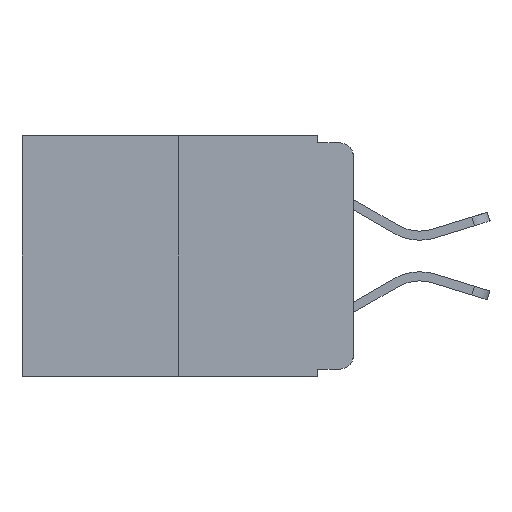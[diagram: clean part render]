
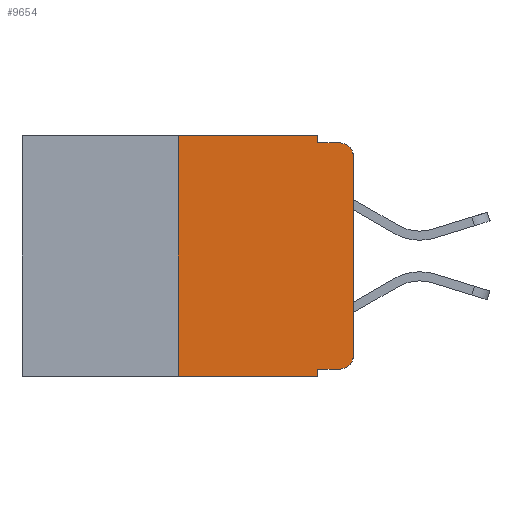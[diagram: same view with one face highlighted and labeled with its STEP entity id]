
A CAD part, left-side view. The second image highlights one B-rep face of the part: STEP entity #9654.
In plain terms, the highlighted planar face has unit normal (-1, 0, 0).
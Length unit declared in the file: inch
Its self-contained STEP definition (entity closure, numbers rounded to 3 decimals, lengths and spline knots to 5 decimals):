
#109 = ORIENTED_EDGE ( 'NONE', *, *, #12100, .F. ) ;
#621 = ORIENTED_EDGE ( 'NONE', *, *, #23641, .F. ) ;
#815 = LINE ( 'NONE', #3153, #20072 ) ;
#1207 = ORIENTED_EDGE ( 'NONE', *, *, #16410, .F. ) ;
#1382 = ORIENTED_EDGE ( 'NONE', *, *, #4426, .T. ) ;
#1397 = CARTESIAN_POINT ( 'NONE',  ( 0., 0.02, -0.03 ) ) ;
#1528 = CARTESIAN_POINT ( 'NONE',  ( 0., 0.051, -0.01 ) ) ;
#1575 = PLANE ( 'NONE',  #7291 ) ;
#1673 = ORIENTED_EDGE ( 'NONE', *, *, #8745, .F. ) ;
#1762 = CIRCLE ( 'NONE', #21992, 0.02 ) ;
#1882 = VECTOR ( 'NONE', #16348, 39.37008 ) ;
#2159 = ORIENTED_EDGE ( 'NONE', *, *, #24383, .T. ) ;
#2772 = ORIENTED_EDGE ( 'NONE', *, *, #15615, .T. ) ;
#3153 = CARTESIAN_POINT ( 'NONE',  ( 0., 0., 0. ) ) ;
#3206 = LINE ( 'NONE', #22989, #22865 ) ;
#3337 = ORIENTED_EDGE ( 'NONE', *, *, #15472, .T. ) ;
#3418 = DIRECTION ( 'NONE',  ( 0., 0., -1. ) ) ;
#3489 = ORIENTED_EDGE ( 'NONE', *, *, #11644, .T. ) ;
#4426 = EDGE_CURVE ( 'NONE', #17896, #7788, #3206, .T. ) ;
#4738 = DIRECTION ( 'NONE',  ( 0., 0., -1. ) ) ;
#5525 = CARTESIAN_POINT ( 'NONE',  ( 0., 0.473, 0. ) ) ;
#5597 = VERTEX_POINT ( 'NONE', #15322 ) ;
#6292 = VERTEX_POINT ( 'NONE', #21320 ) ;
#7291 = AXIS2_PLACEMENT_3D ( 'NONE', #5525, #24467, #13225 ) ;
#7560 = CARTESIAN_POINT ( 'NONE',  ( 0., 0.473, 0. ) ) ;
#7784 = LINE ( 'NONE', #8621, #17892 ) ;
#7788 = VERTEX_POINT ( 'NONE', #19120 ) ;
#7796 = EDGE_CURVE ( 'NONE', #18783, #20367, #13653, .T. ) ;
#7810 = CARTESIAN_POINT ( 'NONE',  ( 0., 0.051, -0.01 ) ) ;
#8621 = CARTESIAN_POINT ( 'NONE',  ( 0., 0.051, 0. ) ) ;
#8745 = EDGE_CURVE ( 'NONE', #5597, #7788, #17229, .T. ) ;
#9654 = ADVANCED_FACE ( 'NONE', ( #13890 ), #1575, .F. ) ;
#9754 = CARTESIAN_POINT ( 'NONE',  ( 0., 0.02, -0.313 ) ) ;
#9822 = DIRECTION ( 'NONE',  ( 0., -1., 0. ) ) ;
#9935 = EDGE_LOOP ( 'NONE', ( #3337, #3489, #10934, #109, #621, #1207, #1382, #1673, #2159, #2772 ) ) ;
#10069 = CARTESIAN_POINT ( 'NONE',  ( 0., 0.02, -0.01 ) ) ;
#10619 = CARTESIAN_POINT ( 'NONE',  ( 0., 0.051, 0. ) ) ;
#10934 = ORIENTED_EDGE ( 'NONE', *, *, #7796, .F. ) ;
#11644 = EDGE_CURVE ( 'NONE', #23990, #20367, #18529, .T. ) ;
#11646 = DIRECTION ( 'NONE',  ( 0., 0., -1. ) ) ;
#11850 = VECTOR ( 'NONE', #20224, 39.37008 ) ;
#12008 = DIRECTION ( 'NONE',  ( 0., 0., 1. ) ) ;
#12100 = EDGE_CURVE ( 'NONE', #13400, #18783, #7784, .T. ) ;
#13100 = CARTESIAN_POINT ( 'NONE',  ( 0., 0.25, -0.343 ) ) ;
#13225 = DIRECTION ( 'NONE',  ( 0., 0., -1. ) ) ;
#13342 = CARTESIAN_POINT ( 'NONE',  ( 0., 0., -0.313 ) ) ;
#13400 = VERTEX_POINT ( 'NONE', #24643 ) ;
#13653 = LINE ( 'NONE', #7810, #18726 ) ;
#13678 = CARTESIAN_POINT ( 'NONE',  ( 0., 0.02, -0.333 ) ) ;
#13890 = FACE_OUTER_BOUND ( 'NONE', #9935, .T. ) ;
#14921 = DIRECTION ( 'NONE',  ( -1., 0., 0. ) ) ;
#15172 = VECTOR ( 'NONE', #12008, 39.37008 ) ;
#15322 = CARTESIAN_POINT ( 'NONE',  ( 0., 0.051, -0.333 ) ) ;
#15472 = EDGE_CURVE ( 'NONE', #17935, #23990, #815, .T. ) ;
#15615 = EDGE_CURVE ( 'NONE', #16353, #17935, #1762, .T. ) ;
#16348 = DIRECTION ( 'NONE',  ( 0., 0., -1. ) ) ;
#16353 = VERTEX_POINT ( 'NONE', #13678 ) ;
#16410 = EDGE_CURVE ( 'NONE', #17896, #6292, #20196, .T. ) ;
#17146 = DIRECTION ( 'NONE',  ( 0., -1., 0. ) ) ;
#17229 = LINE ( 'NONE', #10619, #1882 ) ;
#17653 = CARTESIAN_POINT ( 'NONE',  ( 0., 0.25, 0. ) ) ;
#17892 = VECTOR ( 'NONE', #4738, 39.37008 ) ;
#17896 = VERTEX_POINT ( 'NONE', #13100 ) ;
#17935 = VERTEX_POINT ( 'NONE', #13342 ) ;
#18327 = CARTESIAN_POINT ( 'NONE',  ( 0., 0.051, -0.333 ) ) ;
#18401 = DIRECTION ( 'NONE',  ( 0., 0., 1. ) ) ;
#18429 = VECTOR ( 'NONE', #17146, 39.37008 ) ;
#18529 = CIRCLE ( 'NONE', #24716, 0.02 ) ;
#18726 = VECTOR ( 'NONE', #21104, 39.37008 ) ;
#18783 = VERTEX_POINT ( 'NONE', #1528 ) ;
#19120 = CARTESIAN_POINT ( 'NONE',  ( 0., 0.051, -0.343 ) ) ;
#20072 = VECTOR ( 'NONE', #18401, 39.37008 ) ;
#20196 = LINE ( 'NONE', #17653, #15172 ) ;
#20224 = DIRECTION ( 'NONE',  ( 0., -1., 0. ) ) ;
#20367 = VERTEX_POINT ( 'NONE', #10069 ) ;
#21104 = DIRECTION ( 'NONE',  ( 0., -1., 0. ) ) ;
#21320 = CARTESIAN_POINT ( 'NONE',  ( 0., 0.25, 0. ) ) ;
#21952 = CARTESIAN_POINT ( 'NONE',  ( 0., 0., -0.03 ) ) ;
#21992 = AXIS2_PLACEMENT_3D ( 'NONE', #9754, #22931, #11646 ) ;
#22494 = LINE ( 'NONE', #18327, #11850 ) ;
#22865 = VECTOR ( 'NONE', #9822, 39.37008 ) ;
#22931 = DIRECTION ( 'NONE',  ( -1., 0., 0. ) ) ;
#22989 = CARTESIAN_POINT ( 'NONE',  ( 0., 0.473, -0.343 ) ) ;
#23641 = EDGE_CURVE ( 'NONE', #6292, #13400, #23947, .T. ) ;
#23947 = LINE ( 'NONE', #7560, #18429 ) ;
#23990 = VERTEX_POINT ( 'NONE', #21952 ) ;
#24383 = EDGE_CURVE ( 'NONE', #5597, #16353, #22494, .T. ) ;
#24467 = DIRECTION ( 'NONE',  ( 1., 0., 0. ) ) ;
#24643 = CARTESIAN_POINT ( 'NONE',  ( 0., 0.051, 0. ) ) ;
#24716 = AXIS2_PLACEMENT_3D ( 'NONE', #1397, #14921, #3418 ) ;
